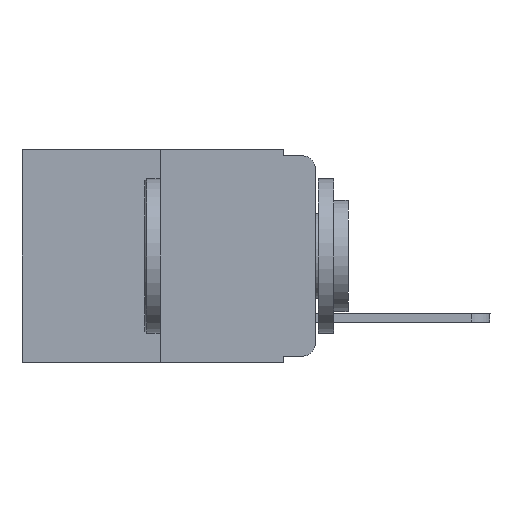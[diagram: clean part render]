
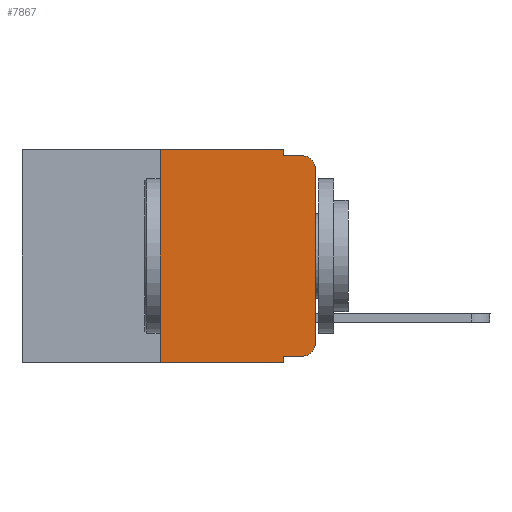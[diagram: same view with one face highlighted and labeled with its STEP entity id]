
A CAD part, left-side view. The second image highlights one B-rep face of the part: STEP entity #7867.
In plain terms, the highlighted planar face has unit normal (-1, 0, 0).
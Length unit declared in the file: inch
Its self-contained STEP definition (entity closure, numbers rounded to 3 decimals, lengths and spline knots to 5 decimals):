
#558 = DIRECTION ( 'NONE',  ( 0., -1., 0. ) ) ;
#946 = DIRECTION ( 'NONE',  ( -1., 0., 0. ) ) ;
#1053 = VERTEX_POINT ( 'NONE', #6468 ) ;
#1179 = LINE ( 'NONE', #8275, #14489 ) ;
#1187 = ORIENTED_EDGE ( 'NONE', *, *, #4659, .F. ) ;
#1307 = VECTOR ( 'NONE', #558, 39.37008 ) ;
#1466 = EDGE_CURVE ( 'NONE', #4116, #14905, #10980, .T. ) ;
#1582 = CARTESIAN_POINT ( 'NONE',  ( 0., 0.02, -0.01 ) ) ;
#1777 = EDGE_CURVE ( 'NONE', #5297, #6471, #1179, .T. ) ;
#2160 = ORIENTED_EDGE ( 'NONE', *, *, #1777, .T. ) ;
#2380 = DIRECTION ( 'NONE',  ( 0., -1., 0. ) ) ;
#2625 = AXIS2_PLACEMENT_3D ( 'NONE', #11495, #5756, #10307 ) ;
#2764 = VECTOR ( 'NONE', #6507, 39.37008 ) ;
#2895 = VECTOR ( 'NONE', #3184, 39.37008 ) ;
#2937 = EDGE_CURVE ( 'NONE', #7926, #7995, #11551, .T. ) ;
#3184 = DIRECTION ( 'NONE',  ( 0., 0., -1. ) ) ;
#3523 = AXIS2_PLACEMENT_3D ( 'NONE', #10580, #946, #7960 ) ;
#3532 = ORIENTED_EDGE ( 'NONE', *, *, #15138, .F. ) ;
#3630 = EDGE_LOOP ( 'NONE', ( #6999, #15376, #13340, #3532, #1187, #9741, #13631, #13957, #2160, #14705 ) ) ;
#4116 = VERTEX_POINT ( 'NONE', #12137 ) ;
#4120 = LINE ( 'NONE', #7869, #15090 ) ;
#4208 = CARTESIAN_POINT ( 'NONE',  ( 0., 0.051, 0. ) ) ;
#4308 = EDGE_CURVE ( 'NONE', #14905, #8989, #7696, .T. ) ;
#4659 = EDGE_CURVE ( 'NONE', #1053, #6409, #7505, .T. ) ;
#4673 = DIRECTION ( 'NONE',  ( 1., 0., 0. ) ) ;
#4705 = AXIS2_PLACEMENT_3D ( 'NONE', #15610, #4673, #11845 ) ;
#4887 = CARTESIAN_POINT ( 'NONE',  ( 0., 0.051, -0.01 ) ) ;
#5104 = CARTESIAN_POINT ( 'NONE',  ( 0., 0.473, 0. ) ) ;
#5286 = EDGE_CURVE ( 'NONE', #5297, #7995, #7874, .T. ) ;
#5297 = VERTEX_POINT ( 'NONE', #10881 ) ;
#5756 = DIRECTION ( 'NONE',  ( -1., 0., 0. ) ) ;
#5795 = PLANE ( 'NONE',  #4705 ) ;
#5973 = DIRECTION ( 'NONE',  ( 0., 0., -1. ) ) ;
#6409 = VERTEX_POINT ( 'NONE', #12983 ) ;
#6434 = VECTOR ( 'NONE', #14744, 39.37008 ) ;
#6468 = CARTESIAN_POINT ( 'NONE',  ( 0., 0.25, 0. ) ) ;
#6471 = VERTEX_POINT ( 'NONE', #7966 ) ;
#6507 = DIRECTION ( 'NONE',  ( 0., 0., 1. ) ) ;
#6680 = DIRECTION ( 'NONE',  ( 0., -1., 0. ) ) ;
#6999 = ORIENTED_EDGE ( 'NONE', *, *, #1466, .T. ) ;
#7505 = LINE ( 'NONE', #5104, #9745 ) ;
#7696 = CIRCLE ( 'NONE', #2625, 0.02 ) ;
#7846 = CIRCLE ( 'NONE', #3523, 0.02 ) ;
#7867 = ADVANCED_FACE ( 'NONE', ( #9609 ), #5795, .F. ) ;
#7869 = CARTESIAN_POINT ( 'NONE',  ( 0., 0.051, -0.01 ) ) ;
#7874 = LINE ( 'NONE', #4208, #2895 ) ;
#7926 = VERTEX_POINT ( 'NONE', #12377 ) ;
#7960 = DIRECTION ( 'NONE',  ( 0., 0., -1. ) ) ;
#7966 = CARTESIAN_POINT ( 'NONE',  ( 0., 0.02, -0.333 ) ) ;
#7995 = VERTEX_POINT ( 'NONE', #10140 ) ;
#8275 = CARTESIAN_POINT ( 'NONE',  ( 0., 0.051, -0.333 ) ) ;
#8581 = CARTESIAN_POINT ( 'NONE',  ( 0., 0.051, 0. ) ) ;
#8735 = CARTESIAN_POINT ( 'NONE',  ( 0., 0.25, 0. ) ) ;
#8917 = CARTESIAN_POINT ( 'NONE',  ( 0., 0., -0.03 ) ) ;
#8989 = VERTEX_POINT ( 'NONE', #1582 ) ;
#9609 = FACE_OUTER_BOUND ( 'NONE', #3630, .T. ) ;
#9741 = ORIENTED_EDGE ( 'NONE', *, *, #10762, .F. ) ;
#9745 = VECTOR ( 'NONE', #12514, 39.37008 ) ;
#9799 = VERTEX_POINT ( 'NONE', #4887 ) ;
#10140 = CARTESIAN_POINT ( 'NONE',  ( 0., 0.051, -0.343 ) ) ;
#10307 = DIRECTION ( 'NONE',  ( 0., 0., -1. ) ) ;
#10475 = VECTOR ( 'NONE', #5973, 39.37008 ) ;
#10513 = EDGE_CURVE ( 'NONE', #6471, #4116, #7846, .T. ) ;
#10580 = CARTESIAN_POINT ( 'NONE',  ( 0., 0.02, -0.313 ) ) ;
#10762 = EDGE_CURVE ( 'NONE', #7926, #1053, #11192, .T. ) ;
#10881 = CARTESIAN_POINT ( 'NONE',  ( 0., 0.051, -0.333 ) ) ;
#10980 = LINE ( 'NONE', #14823, #6434 ) ;
#11192 = LINE ( 'NONE', #8735, #2764 ) ;
#11495 = CARTESIAN_POINT ( 'NONE',  ( 0., 0.02, -0.03 ) ) ;
#11551 = LINE ( 'NONE', #14117, #1307 ) ;
#11845 = DIRECTION ( 'NONE',  ( 0., 0., -1. ) ) ;
#12137 = CARTESIAN_POINT ( 'NONE',  ( 0., 0., -0.313 ) ) ;
#12170 = LINE ( 'NONE', #8581, #10475 ) ;
#12377 = CARTESIAN_POINT ( 'NONE',  ( 0., 0.25, -0.343 ) ) ;
#12514 = DIRECTION ( 'NONE',  ( 0., -1., 0. ) ) ;
#12983 = CARTESIAN_POINT ( 'NONE',  ( 0., 0.051, 0. ) ) ;
#13340 = ORIENTED_EDGE ( 'NONE', *, *, #15386, .F. ) ;
#13631 = ORIENTED_EDGE ( 'NONE', *, *, #2937, .T. ) ;
#13957 = ORIENTED_EDGE ( 'NONE', *, *, #5286, .F. ) ;
#14117 = CARTESIAN_POINT ( 'NONE',  ( 0., 0.473, -0.343 ) ) ;
#14489 = VECTOR ( 'NONE', #2380, 39.37008 ) ;
#14705 = ORIENTED_EDGE ( 'NONE', *, *, #10513, .T. ) ;
#14744 = DIRECTION ( 'NONE',  ( 0., 0., 1. ) ) ;
#14823 = CARTESIAN_POINT ( 'NONE',  ( 0., 0., 0. ) ) ;
#14905 = VERTEX_POINT ( 'NONE', #8917 ) ;
#15090 = VECTOR ( 'NONE', #6680, 39.37008 ) ;
#15138 = EDGE_CURVE ( 'NONE', #6409, #9799, #12170, .T. ) ;
#15376 = ORIENTED_EDGE ( 'NONE', *, *, #4308, .T. ) ;
#15386 = EDGE_CURVE ( 'NONE', #9799, #8989, #4120, .T. ) ;
#15610 = CARTESIAN_POINT ( 'NONE',  ( 0., 0.473, 0. ) ) ;
